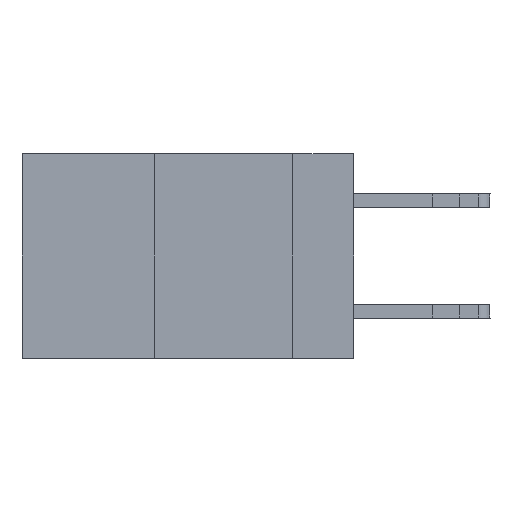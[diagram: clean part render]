
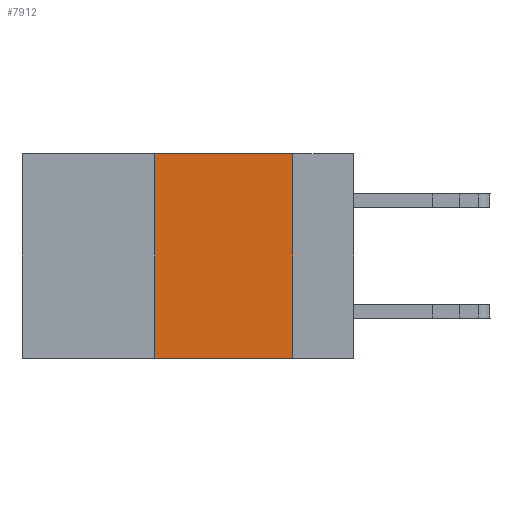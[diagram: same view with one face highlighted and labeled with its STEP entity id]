
A CAD part, left-side view. The second image highlights one B-rep face of the part: STEP entity #7912.
In plain terms, the highlighted planar face has unit normal (-1, 0, 0).
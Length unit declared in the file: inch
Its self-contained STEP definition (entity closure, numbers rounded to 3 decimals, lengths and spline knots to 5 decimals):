
#1688 = EDGE_CURVE ( 'NONE', #28418, #34243, #33268, .T. ) ;
#1828 = FACE_OUTER_BOUND ( 'NONE', #22286, .T. ) ;
#3625 = VECTOR ( 'NONE', #22478, 39.37008 ) ;
#4152 = EDGE_CURVE ( 'NONE', #9275, #34243, #7983, .T. ) ;
#4335 = CARTESIAN_POINT ( 'NONE',  ( 0., 0.6, 0. ) ) ;
#4702 = CARTESIAN_POINT ( 'NONE',  ( 0., 0.11, 0. ) ) ;
#5835 = ORIENTED_EDGE ( 'NONE', *, *, #4152, .T. ) ;
#7912 = ADVANCED_FACE ( 'NONE', ( #1828 ), #15821, .F. ) ;
#7983 = LINE ( 'NONE', #10954, #24366 ) ;
#8053 = ORIENTED_EDGE ( 'NONE', *, *, #1688, .F. ) ;
#8251 = LINE ( 'NONE', #10042, #22305 ) ;
#9275 = VERTEX_POINT ( 'NONE', #24104 ) ;
#10042 = CARTESIAN_POINT ( 'NONE',  ( 0., 0.36, 0. ) ) ;
#10244 = DIRECTION ( 'NONE',  ( 1., 0., 0. ) ) ;
#10954 = CARTESIAN_POINT ( 'NONE',  ( 0., 0.6, -0.37 ) ) ;
#12259 = DIRECTION ( 'NONE',  ( 0., 0., -1. ) ) ;
#12456 = EDGE_CURVE ( 'NONE', #9275, #30463, #8251, .T. ) ;
#13237 = DIRECTION ( 'NONE',  ( 0., 0., -1. ) ) ;
#14172 = DIRECTION ( 'NONE',  ( 0., -1., 0. ) ) ;
#15821 = PLANE ( 'NONE',  #38232 ) ;
#16427 = CARTESIAN_POINT ( 'NONE',  ( 0., 0.11, -0.37 ) ) ;
#17885 = ORIENTED_EDGE ( 'NONE', *, *, #38718, .F. ) ;
#19554 = LINE ( 'NONE', #31245, #3625 ) ;
#21939 = VECTOR ( 'NONE', #12259, 39.37008 ) ;
#22286 = EDGE_LOOP ( 'NONE', ( #8053, #17885, #28731, #5835 ) ) ;
#22305 = VECTOR ( 'NONE', #27935, 39.37008 ) ;
#22478 = DIRECTION ( 'NONE',  ( 0., -1., 0. ) ) ;
#24104 = CARTESIAN_POINT ( 'NONE',  ( 0., 0.36, -0.37 ) ) ;
#24366 = VECTOR ( 'NONE', #14172, 39.37008 ) ;
#27935 = DIRECTION ( 'NONE',  ( 0., 0., 1. ) ) ;
#28418 = VERTEX_POINT ( 'NONE', #4702 ) ;
#28731 = ORIENTED_EDGE ( 'NONE', *, *, #12456, .F. ) ;
#29866 = CARTESIAN_POINT ( 'NONE',  ( 0., 0.36, 0. ) ) ;
#30463 = VERTEX_POINT ( 'NONE', #29866 ) ;
#31245 = CARTESIAN_POINT ( 'NONE',  ( 0., 0.6, 0. ) ) ;
#33268 = LINE ( 'NONE', #33428, #21939 ) ;
#33428 = CARTESIAN_POINT ( 'NONE',  ( 0., 0.11, 0. ) ) ;
#34243 = VERTEX_POINT ( 'NONE', #16427 ) ;
#38232 = AXIS2_PLACEMENT_3D ( 'NONE', #4335, #10244, #13237 ) ;
#38718 = EDGE_CURVE ( 'NONE', #30463, #28418, #19554, .T. ) ;
